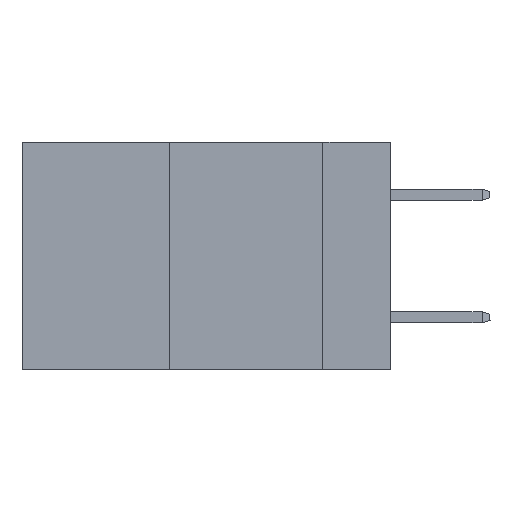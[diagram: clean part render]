
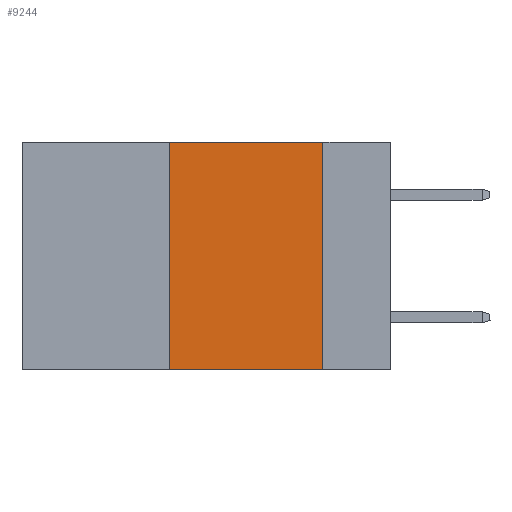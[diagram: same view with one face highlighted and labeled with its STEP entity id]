
A CAD part, left-side view. The second image highlights one B-rep face of the part: STEP entity #9244.
In plain terms, the highlighted planar face has unit normal (-1, 0, 0).
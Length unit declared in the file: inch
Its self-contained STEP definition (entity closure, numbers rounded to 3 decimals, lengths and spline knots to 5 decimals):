
#70 = DIRECTION ( 'NONE',  ( 0., -1., 0. ) ) ;
#1052 = CARTESIAN_POINT ( 'NONE',  ( 0., 0.36, 0. ) ) ;
#1879 = VECTOR ( 'NONE', #7151, 39.37008 ) ;
#2503 = EDGE_CURVE ( 'NONE', #39861, #36688, #2871, .T. ) ;
#2716 = ORIENTED_EDGE ( 'NONE', *, *, #9898, .F. ) ;
#2778 = CARTESIAN_POINT ( 'NONE',  ( 0., 0.6, 0. ) ) ;
#2871 = LINE ( 'NONE', #32482, #32117 ) ;
#2917 = EDGE_CURVE ( 'NONE', #23564, #39861, #8695, .T. ) ;
#3339 = CARTESIAN_POINT ( 'NONE',  ( 0., 0.6, -0.37 ) ) ;
#3898 = CARTESIAN_POINT ( 'NONE',  ( 0., 0.36, 0. ) ) ;
#4235 = LINE ( 'NONE', #3339, #23189 ) ;
#5298 = VECTOR ( 'NONE', #22546, 39.37008 ) ;
#5902 = DIRECTION ( 'NONE',  ( 0., 0., -1. ) ) ;
#7151 = DIRECTION ( 'NONE',  ( 0., -1., 0. ) ) ;
#7194 = AXIS2_PLACEMENT_3D ( 'NONE', #2778, #24516, #5902 ) ;
#8695 = LINE ( 'NONE', #31504, #1879 ) ;
#9244 = ADVANCED_FACE ( 'NONE', ( #21355 ), #21384, .F. ) ;
#9597 = VERTEX_POINT ( 'NONE', #17522 ) ;
#9898 = EDGE_CURVE ( 'NONE', #9597, #23564, #37413, .T. ) ;
#11639 = DIRECTION ( 'NONE',  ( 0., 0., -1. ) ) ;
#12222 = ORIENTED_EDGE ( 'NONE', *, *, #2503, .F. ) ;
#12307 = CARTESIAN_POINT ( 'NONE',  ( 0., 0.11, 0. ) ) ;
#15792 = EDGE_LOOP ( 'NONE', ( #12222, #35374, #2716, #16056 ) ) ;
#16056 = ORIENTED_EDGE ( 'NONE', *, *, #25590, .T. ) ;
#17522 = CARTESIAN_POINT ( 'NONE',  ( 0., 0.36, -0.37 ) ) ;
#21355 = FACE_OUTER_BOUND ( 'NONE', #15792, .T. ) ;
#21384 = PLANE ( 'NONE',  #7194 ) ;
#22546 = DIRECTION ( 'NONE',  ( 0., 0., 1. ) ) ;
#23189 = VECTOR ( 'NONE', #70, 39.37008 ) ;
#23564 = VERTEX_POINT ( 'NONE', #3898 ) ;
#24516 = DIRECTION ( 'NONE',  ( 1., 0., 0. ) ) ;
#25590 = EDGE_CURVE ( 'NONE', #9597, #36688, #4235, .T. ) ;
#31504 = CARTESIAN_POINT ( 'NONE',  ( 0., 0.6, 0. ) ) ;
#32117 = VECTOR ( 'NONE', #11639, 39.37008 ) ;
#32482 = CARTESIAN_POINT ( 'NONE',  ( 0., 0.11, 0. ) ) ;
#35374 = ORIENTED_EDGE ( 'NONE', *, *, #2917, .F. ) ;
#36688 = VERTEX_POINT ( 'NONE', #38151 ) ;
#37413 = LINE ( 'NONE', #1052, #5298 ) ;
#38151 = CARTESIAN_POINT ( 'NONE',  ( 0., 0.11, -0.37 ) ) ;
#39861 = VERTEX_POINT ( 'NONE', #12307 ) ;
